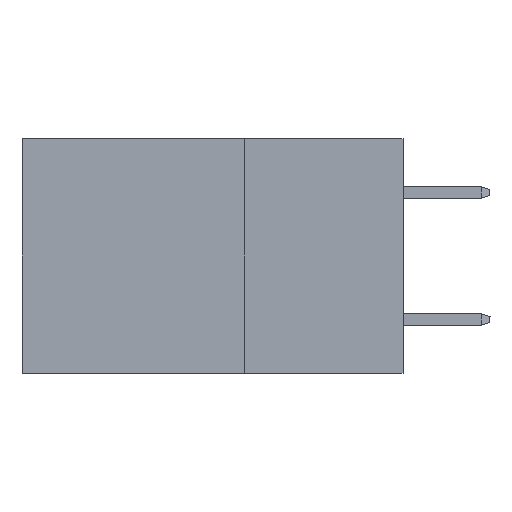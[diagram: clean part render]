
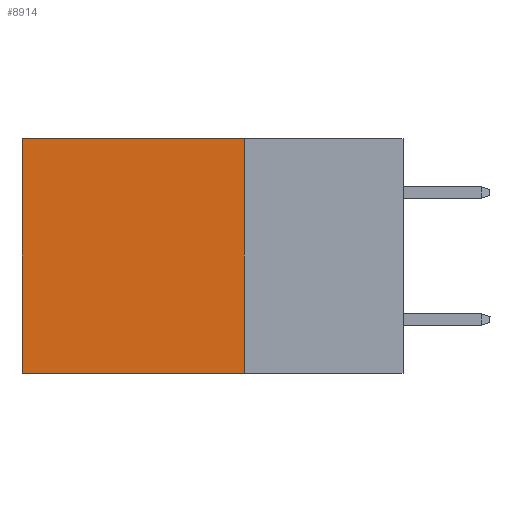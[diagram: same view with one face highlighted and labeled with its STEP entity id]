
A CAD part, left-side view. The second image highlights one B-rep face of the part: STEP entity #8914.
In plain terms, the highlighted planar face has unit normal (-1, 0, 0).
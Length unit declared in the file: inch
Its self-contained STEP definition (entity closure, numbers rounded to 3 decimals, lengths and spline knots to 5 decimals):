
#21 = LINE ( 'NONE', #7942, #2324 ) ;
#602 = EDGE_LOOP ( 'NONE', ( #7826, #4141, #8245, #2091 ) ) ;
#821 = DIRECTION ( 'NONE',  ( 0., 0., -1. ) ) ;
#1245 = CARTESIAN_POINT ( 'NONE',  ( 0.2875, 0.6, 0. ) ) ;
#1297 = LINE ( 'NONE', #3767, #4655 ) ;
#1839 = CARTESIAN_POINT ( 'NONE',  ( 0.2875, 0.6, 0. ) ) ;
#1969 = CARTESIAN_POINT ( 'NONE',  ( 0.2875, 0.25, 0. ) ) ;
#2091 = ORIENTED_EDGE ( 'NONE', *, *, #3584, .T. ) ;
#2324 = VECTOR ( 'NONE', #821, 39.37008 ) ;
#2372 = VERTEX_POINT ( 'NONE', #1839 ) ;
#2735 = VERTEX_POINT ( 'NONE', #6564 ) ;
#2866 = FACE_OUTER_BOUND ( 'NONE', #602, .T. ) ;
#3584 = EDGE_CURVE ( 'NONE', #6077, #2372, #7398, .T. ) ;
#3767 = CARTESIAN_POINT ( 'NONE',  ( 0.2875, 0.25, -0.37 ) ) ;
#3796 = EDGE_CURVE ( 'NONE', #6077, #2735, #21, .T. ) ;
#4141 = ORIENTED_EDGE ( 'NONE', *, *, #6003, .F. ) ;
#4655 = VECTOR ( 'NONE', #9952, 39.37008 ) ;
#4720 = EDGE_CURVE ( 'NONE', #2372, #6703, #10002, .T. ) ;
#5219 = PLANE ( 'NONE',  #8497 ) ;
#5266 = CARTESIAN_POINT ( 'NONE',  ( 0.2875, 0.25, 0. ) ) ;
#6003 = EDGE_CURVE ( 'NONE', #2735, #6703, #1297, .T. ) ;
#6077 = VERTEX_POINT ( 'NONE', #6509 ) ;
#6140 = DIRECTION ( 'NONE',  ( 0., 0., -1. ) ) ;
#6287 = VECTOR ( 'NONE', #7604, 39.37008 ) ;
#6429 = VECTOR ( 'NONE', #6617, 39.37008 ) ;
#6509 = CARTESIAN_POINT ( 'NONE',  ( 0.2875, 0.25, 0. ) ) ;
#6564 = CARTESIAN_POINT ( 'NONE',  ( 0.2875, 0.25, -0.37 ) ) ;
#6617 = DIRECTION ( 'NONE',  ( 0., 1., 0. ) ) ;
#6703 = VERTEX_POINT ( 'NONE', #7002 ) ;
#7002 = CARTESIAN_POINT ( 'NONE',  ( 0.2875, 0.6, -0.37 ) ) ;
#7398 = LINE ( 'NONE', #1969, #6429 ) ;
#7604 = DIRECTION ( 'NONE',  ( 0., 0., -1. ) ) ;
#7826 = ORIENTED_EDGE ( 'NONE', *, *, #4720, .T. ) ;
#7942 = CARTESIAN_POINT ( 'NONE',  ( 0.2875, 0.25, 0. ) ) ;
#8245 = ORIENTED_EDGE ( 'NONE', *, *, #3796, .F. ) ;
#8497 = AXIS2_PLACEMENT_3D ( 'NONE', #5266, #9993, #6140 ) ;
#8914 = ADVANCED_FACE ( 'NONE', ( #2866 ), #5219, .F. ) ;
#9952 = DIRECTION ( 'NONE',  ( 0., 1., 0. ) ) ;
#9993 = DIRECTION ( 'NONE',  ( 1., 0., 0. ) ) ;
#10002 = LINE ( 'NONE', #1245, #6287 ) ;
